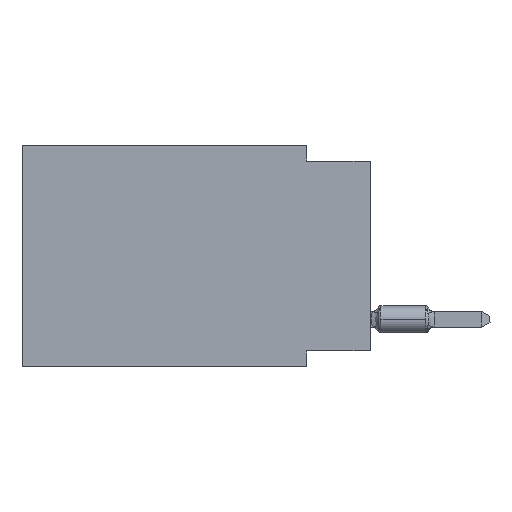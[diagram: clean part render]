
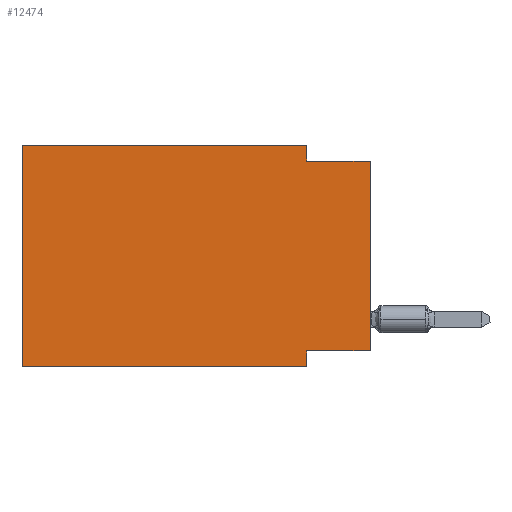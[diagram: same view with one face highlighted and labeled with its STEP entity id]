
A CAD part, left-side view. The second image highlights one B-rep face of the part: STEP entity #12474.
In plain terms, the highlighted planar face has unit normal (-1, 0, 0).
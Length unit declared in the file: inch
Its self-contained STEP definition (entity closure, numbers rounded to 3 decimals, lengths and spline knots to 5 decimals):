
#108 = CARTESIAN_POINT ( 'NONE',  ( 0., 0., -0.025 ) ) ;
#123 = VERTEX_POINT ( 'NONE', #4933 ) ;
#440 = VERTEX_POINT ( 'NONE', #4794 ) ;
#586 = CARTESIAN_POINT ( 'NONE',  ( 0., 0.55, 0. ) ) ;
#856 = ORIENTED_EDGE ( 'NONE', *, *, #12096, .F. ) ;
#904 = VECTOR ( 'NONE', #10197, 39.37008 ) ;
#1099 = LINE ( 'NONE', #8760, #9781 ) ;
#1341 = EDGE_CURVE ( 'NONE', #5314, #13516, #3290, .T. ) ;
#1402 = ORIENTED_EDGE ( 'NONE', *, *, #14268, .F. ) ;
#1686 = DIRECTION ( 'NONE',  ( 0., -1., 0. ) ) ;
#2185 = CARTESIAN_POINT ( 'NONE',  ( 0., 0.1, -0.025 ) ) ;
#2357 = DIRECTION ( 'NONE',  ( 0., 0., 1. ) ) ;
#2555 = EDGE_CURVE ( 'NONE', #5213, #123, #4738, .T. ) ;
#2892 = LINE ( 'NONE', #13896, #11795 ) ;
#2917 = CARTESIAN_POINT ( 'NONE',  ( 0., 0.1, 0. ) ) ;
#3290 = LINE ( 'NONE', #13583, #904 ) ;
#4487 = LINE ( 'NONE', #11763, #8033 ) ;
#4738 = LINE ( 'NONE', #13552, #5841 ) ;
#4744 = LINE ( 'NONE', #7063, #6227 ) ;
#4794 = CARTESIAN_POINT ( 'NONE',  ( 0., 0., -0.325 ) ) ;
#4933 = CARTESIAN_POINT ( 'NONE',  ( 0., 0.1, -0.35 ) ) ;
#4999 = VERTEX_POINT ( 'NONE', #8156 ) ;
#5065 = ORIENTED_EDGE ( 'NONE', *, *, #6028, .F. ) ;
#5097 = ORIENTED_EDGE ( 'NONE', *, *, #15289, .F. ) ;
#5109 = VECTOR ( 'NONE', #7238, 39.37008 ) ;
#5213 = VERTEX_POINT ( 'NONE', #13256 ) ;
#5314 = VERTEX_POINT ( 'NONE', #2917 ) ;
#5841 = VECTOR ( 'NONE', #6502, 39.37008 ) ;
#5919 = EDGE_CURVE ( 'NONE', #4999, #123, #2892, .T. ) ;
#6028 = EDGE_CURVE ( 'NONE', #5213, #9820, #4744, .T. ) ;
#6227 = VECTOR ( 'NONE', #2357, 39.37008 ) ;
#6502 = DIRECTION ( 'NONE',  ( 0., -1., 0. ) ) ;
#6871 = DIRECTION ( 'NONE',  ( 1., 0., 0. ) ) ;
#6923 = CARTESIAN_POINT ( 'NONE',  ( 0., 0.55, 0. ) ) ;
#7063 = CARTESIAN_POINT ( 'NONE',  ( 0., 0.55, 0. ) ) ;
#7082 = ORIENTED_EDGE ( 'NONE', *, *, #10593, .T. ) ;
#7238 = DIRECTION ( 'NONE',  ( 0., 0., 1. ) ) ;
#8033 = VECTOR ( 'NONE', #10464, 39.37008 ) ;
#8061 = VERTEX_POINT ( 'NONE', #8266 ) ;
#8156 = CARTESIAN_POINT ( 'NONE',  ( 0., 0.1, -0.325 ) ) ;
#8266 = CARTESIAN_POINT ( 'NONE',  ( 0., 0., -0.025 ) ) ;
#8620 = AXIS2_PLACEMENT_3D ( 'NONE', #6923, #6871, #9270 ) ;
#8760 = CARTESIAN_POINT ( 'NONE',  ( 0., 0.55, 0. ) ) ;
#8843 = EDGE_LOOP ( 'NONE', ( #7082, #1402, #12883, #5097, #5065, #12861, #13561, #856 ) ) ;
#9247 = LINE ( 'NONE', #108, #11676 ) ;
#9270 = DIRECTION ( 'NONE',  ( 0., 0., -1. ) ) ;
#9781 = VECTOR ( 'NONE', #1686, 39.37008 ) ;
#9820 = VERTEX_POINT ( 'NONE', #586 ) ;
#10068 = FACE_OUTER_BOUND ( 'NONE', #8843, .T. ) ;
#10197 = DIRECTION ( 'NONE',  ( 0., 0., -1. ) ) ;
#10464 = DIRECTION ( 'NONE',  ( 0., 1., 0. ) ) ;
#10469 = DIRECTION ( 'NONE',  ( 0., 0., -1. ) ) ;
#10593 = EDGE_CURVE ( 'NONE', #440, #8061, #15251, .T. ) ;
#11621 = PLANE ( 'NONE',  #8620 ) ;
#11676 = VECTOR ( 'NONE', #13182, 39.37008 ) ;
#11763 = CARTESIAN_POINT ( 'NONE',  ( 0., 0., -0.325 ) ) ;
#11795 = VECTOR ( 'NONE', #10469, 39.37008 ) ;
#12096 = EDGE_CURVE ( 'NONE', #440, #4999, #4487, .T. ) ;
#12474 = ADVANCED_FACE ( 'NONE', ( #10068 ), #11621, .F. ) ;
#12861 = ORIENTED_EDGE ( 'NONE', *, *, #2555, .T. ) ;
#12883 = ORIENTED_EDGE ( 'NONE', *, *, #1341, .F. ) ;
#13182 = DIRECTION ( 'NONE',  ( 0., -1., 0. ) ) ;
#13256 = CARTESIAN_POINT ( 'NONE',  ( 0., 0.55, -0.35 ) ) ;
#13516 = VERTEX_POINT ( 'NONE', #2185 ) ;
#13552 = CARTESIAN_POINT ( 'NONE',  ( 0., 0.55, -0.35 ) ) ;
#13561 = ORIENTED_EDGE ( 'NONE', *, *, #5919, .F. ) ;
#13583 = CARTESIAN_POINT ( 'NONE',  ( 0., 0.1, 0. ) ) ;
#13896 = CARTESIAN_POINT ( 'NONE',  ( 0., 0.1, -0.35 ) ) ;
#14178 = CARTESIAN_POINT ( 'NONE',  ( 0., 0., 0. ) ) ;
#14268 = EDGE_CURVE ( 'NONE', #13516, #8061, #9247, .T. ) ;
#15251 = LINE ( 'NONE', #14178, #5109 ) ;
#15289 = EDGE_CURVE ( 'NONE', #9820, #5314, #1099, .T. ) ;
